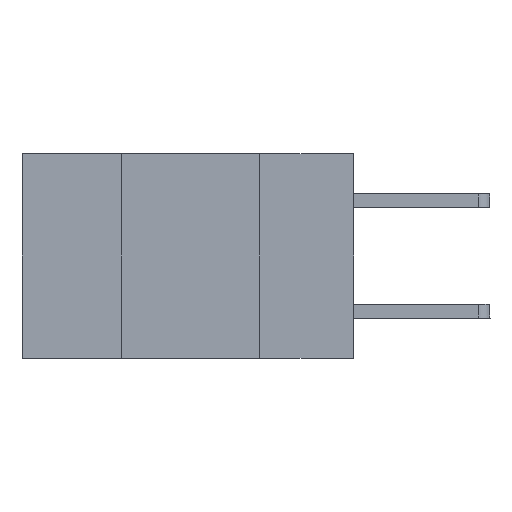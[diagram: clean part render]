
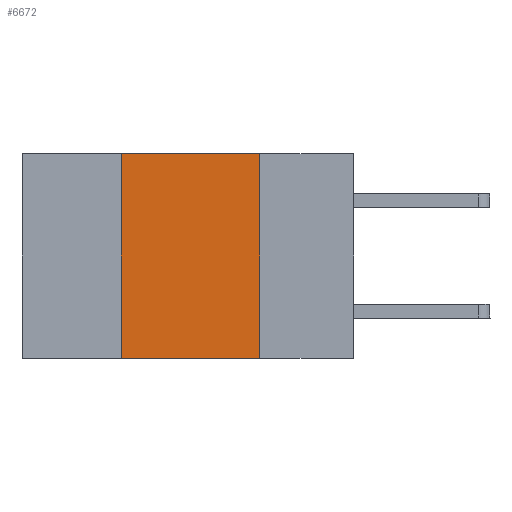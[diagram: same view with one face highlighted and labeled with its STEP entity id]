
A CAD part, left-side view. The second image highlights one B-rep face of the part: STEP entity #6672.
In plain terms, the highlighted planar face has unit normal (-1, 0, 0).
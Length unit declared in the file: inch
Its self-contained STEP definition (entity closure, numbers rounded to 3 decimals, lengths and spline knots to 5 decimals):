
#422 = EDGE_CURVE ( 'NONE', #5106, #916, #1402, .T. ) ;
#471 = CARTESIAN_POINT ( 'NONE',  ( 0., 0.17, 0. ) ) ;
#538 = CARTESIAN_POINT ( 'NONE',  ( 0., 0.17, -0.37 ) ) ;
#916 = VERTEX_POINT ( 'NONE', #5706 ) ;
#1402 = LINE ( 'NONE', #5978, #9259 ) ;
#1543 = LINE ( 'NONE', #9999, #1584 ) ;
#1584 = VECTOR ( 'NONE', #3547, 39.37008 ) ;
#1680 = EDGE_CURVE ( 'NONE', #5106, #8185, #1543, .T. ) ;
#2399 = ORIENTED_EDGE ( 'NONE', *, *, #1680, .T. ) ;
#2403 = CARTESIAN_POINT ( 'NONE',  ( 0., 0.42, -0.37 ) ) ;
#2781 = DIRECTION ( 'NONE',  ( 1., 0., 0. ) ) ;
#3547 = DIRECTION ( 'NONE',  ( 0., -1., 0. ) ) ;
#3837 = ORIENTED_EDGE ( 'NONE', *, *, #10817, .F. ) ;
#3923 = CARTESIAN_POINT ( 'NONE',  ( 0., 0.17, 0. ) ) ;
#4165 = DIRECTION ( 'NONE',  ( 0., 0., 1. ) ) ;
#4503 = DIRECTION ( 'NONE',  ( 0., -1., 0. ) ) ;
#4628 = EDGE_CURVE ( 'NONE', #10243, #8185, #10653, .T. ) ;
#5053 = ORIENTED_EDGE ( 'NONE', *, *, #4628, .F. ) ;
#5106 = VERTEX_POINT ( 'NONE', #2403 ) ;
#5706 = CARTESIAN_POINT ( 'NONE',  ( 0., 0.42, 0. ) ) ;
#5978 = CARTESIAN_POINT ( 'NONE',  ( 0., 0.42, 0. ) ) ;
#6494 = CARTESIAN_POINT ( 'NONE',  ( 0., 0.6, 0. ) ) ;
#6672 = ADVANCED_FACE ( 'NONE', ( #7397 ), #11093, .F. ) ;
#7397 = FACE_OUTER_BOUND ( 'NONE', #9994, .T. ) ;
#7458 = DIRECTION ( 'NONE',  ( 0., 0., -1. ) ) ;
#8185 = VERTEX_POINT ( 'NONE', #538 ) ;
#8847 = DIRECTION ( 'NONE',  ( 0., 0., -1. ) ) ;
#9238 = LINE ( 'NONE', #10985, #9644 ) ;
#9259 = VECTOR ( 'NONE', #4165, 39.37008 ) ;
#9644 = VECTOR ( 'NONE', #4503, 39.37008 ) ;
#9800 = AXIS2_PLACEMENT_3D ( 'NONE', #6494, #2781, #7458 ) ;
#9994 = EDGE_LOOP ( 'NONE', ( #5053, #3837, #10478, #2399 ) ) ;
#9999 = CARTESIAN_POINT ( 'NONE',  ( 0., 0.6, -0.37 ) ) ;
#10243 = VERTEX_POINT ( 'NONE', #3923 ) ;
#10478 = ORIENTED_EDGE ( 'NONE', *, *, #422, .F. ) ;
#10653 = LINE ( 'NONE', #471, #11099 ) ;
#10817 = EDGE_CURVE ( 'NONE', #916, #10243, #9238, .T. ) ;
#10985 = CARTESIAN_POINT ( 'NONE',  ( 0., 0.6, 0. ) ) ;
#11093 = PLANE ( 'NONE',  #9800 ) ;
#11099 = VECTOR ( 'NONE', #8847, 39.37008 ) ;
